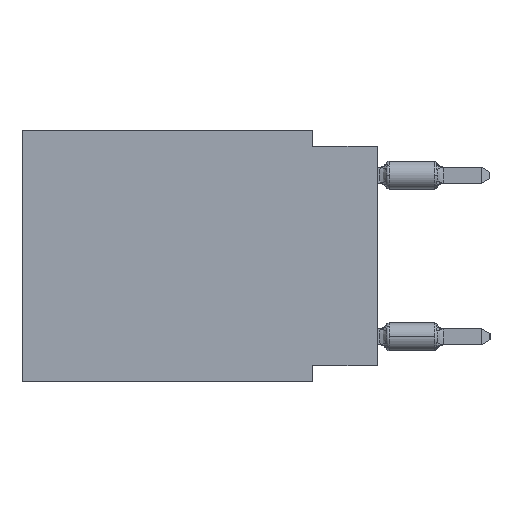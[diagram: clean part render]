
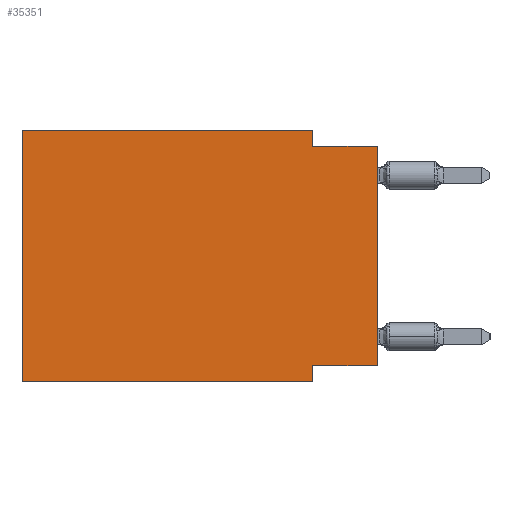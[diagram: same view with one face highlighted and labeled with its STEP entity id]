
A CAD part, left-side view. The second image highlights one B-rep face of the part: STEP entity #35351.
In plain terms, the highlighted planar face has unit normal (-1, 0, 0).
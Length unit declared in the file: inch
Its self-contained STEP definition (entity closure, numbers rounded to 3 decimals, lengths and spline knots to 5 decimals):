
#899 = DIRECTION ( 'NONE',  ( 0., 0., -1. ) ) ;
#2183 = DIRECTION ( 'NONE',  ( 0., 1., 0. ) ) ;
#2944 = VECTOR ( 'NONE', #31111, 39.37008 ) ;
#4536 = VECTOR ( 'NONE', #25142, 39.37008 ) ;
#6134 = LINE ( 'NONE', #20102, #6887 ) ;
#6887 = VECTOR ( 'NONE', #24393, 39.37008 ) ;
#7057 = DIRECTION ( 'NONE',  ( 0., 0., -1. ) ) ;
#7700 = EDGE_CURVE ( 'NONE', #34435, #14014, #41277, .T. ) ;
#8579 = LINE ( 'NONE', #44273, #15129 ) ;
#8936 = CARTESIAN_POINT ( 'NONE',  ( 0., 0., -0.025 ) ) ;
#9552 = VERTEX_POINT ( 'NONE', #8936 ) ;
#10720 = ORIENTED_EDGE ( 'NONE', *, *, #49276, .F. ) ;
#11265 = CARTESIAN_POINT ( 'NONE',  ( 0., 0.1, -0.39 ) ) ;
#11672 = ORIENTED_EDGE ( 'NONE', *, *, #25732, .F. ) ;
#13437 = DIRECTION ( 'NONE',  ( 0., 0., 1. ) ) ;
#13472 = VERTEX_POINT ( 'NONE', #50496 ) ;
#14014 = VERTEX_POINT ( 'NONE', #34338 ) ;
#14554 = CARTESIAN_POINT ( 'NONE',  ( 0., 0.1, 0. ) ) ;
#14652 = LINE ( 'NONE', #14939, #45044 ) ;
#14939 = CARTESIAN_POINT ( 'NONE',  ( 0., 0.55, 0. ) ) ;
#15129 = VECTOR ( 'NONE', #13437, 39.37008 ) ;
#16832 = EDGE_CURVE ( 'NONE', #50899, #9552, #43692, .T. ) ;
#17279 = CARTESIAN_POINT ( 'NONE',  ( 0., 0., -0.365 ) ) ;
#18030 = ORIENTED_EDGE ( 'NONE', *, *, #16832, .F. ) ;
#18857 = DIRECTION ( 'NONE',  ( 1., 0., 0. ) ) ;
#19346 = LINE ( 'NONE', #41317, #32634 ) ;
#20102 = CARTESIAN_POINT ( 'NONE',  ( 0., 0.55, -0.39 ) ) ;
#20781 = EDGE_CURVE ( 'NONE', #14014, #44164, #45247, .T. ) ;
#24393 = DIRECTION ( 'NONE',  ( 0., -1., 0. ) ) ;
#25142 = DIRECTION ( 'NONE',  ( 0., -1., 0. ) ) ;
#25732 = EDGE_CURVE ( 'NONE', #26179, #13472, #44253, .T. ) ;
#25902 = CARTESIAN_POINT ( 'NONE',  ( 0., 0.55, -0.39 ) ) ;
#26179 = VERTEX_POINT ( 'NONE', #25902 ) ;
#27978 = FACE_OUTER_BOUND ( 'NONE', #42163, .T. ) ;
#28060 = DIRECTION ( 'NONE',  ( 0., -1., 0. ) ) ;
#28321 = EDGE_CURVE ( 'NONE', #13472, #35014, #14652, .T. ) ;
#28383 = DIRECTION ( 'NONE',  ( 0., 0., -1. ) ) ;
#28717 = CARTESIAN_POINT ( 'NONE',  ( 0., 0., -0.365 ) ) ;
#29780 = VECTOR ( 'NONE', #2183, 39.37008 ) ;
#31111 = DIRECTION ( 'NONE',  ( 0., 0., 1. ) ) ;
#32634 = VECTOR ( 'NONE', #7057, 39.37008 ) ;
#33953 = ORIENTED_EDGE ( 'NONE', *, *, #44133, .T. ) ;
#34338 = CARTESIAN_POINT ( 'NONE',  ( 0., 0.1, -0.365 ) ) ;
#34435 = VERTEX_POINT ( 'NONE', #17279 ) ;
#35014 = VERTEX_POINT ( 'NONE', #14554 ) ;
#35085 = ORIENTED_EDGE ( 'NONE', *, *, #20781, .F. ) ;
#35351 = ADVANCED_FACE ( 'NONE', ( #27978 ), #44285, .F. ) ;
#38697 = ORIENTED_EDGE ( 'NONE', *, *, #28321, .F. ) ;
#39108 = CARTESIAN_POINT ( 'NONE',  ( 0., 0., -0.025 ) ) ;
#39665 = CARTESIAN_POINT ( 'NONE',  ( 0., 0.55, 0. ) ) ;
#40264 = CARTESIAN_POINT ( 'NONE',  ( 0., 0.55, 0. ) ) ;
#41277 = LINE ( 'NONE', #28717, #29780 ) ;
#41317 = CARTESIAN_POINT ( 'NONE',  ( 0., 0.1, 0. ) ) ;
#42163 = EDGE_LOOP ( 'NONE', ( #48855, #18030, #10720, #38697, #11672, #33953, #35085, #55860 ) ) ;
#43692 = LINE ( 'NONE', #39108, #4536 ) ;
#44133 = EDGE_CURVE ( 'NONE', #26179, #44164, #6134, .T. ) ;
#44164 = VERTEX_POINT ( 'NONE', #11265 ) ;
#44253 = LINE ( 'NONE', #39665, #2944 ) ;
#44273 = CARTESIAN_POINT ( 'NONE',  ( 0., 0., 0. ) ) ;
#44285 = PLANE ( 'NONE',  #53639 ) ;
#44840 = EDGE_CURVE ( 'NONE', #34435, #9552, #8579, .T. ) ;
#45044 = VECTOR ( 'NONE', #28060, 39.37008 ) ;
#45247 = LINE ( 'NONE', #49802, #45771 ) ;
#45771 = VECTOR ( 'NONE', #28383, 39.37008 ) ;
#48855 = ORIENTED_EDGE ( 'NONE', *, *, #44840, .T. ) ;
#49276 = EDGE_CURVE ( 'NONE', #35014, #50899, #19346, .T. ) ;
#49802 = CARTESIAN_POINT ( 'NONE',  ( 0., 0.1, -0.39 ) ) ;
#50496 = CARTESIAN_POINT ( 'NONE',  ( 0., 0.55, 0. ) ) ;
#50641 = CARTESIAN_POINT ( 'NONE',  ( 0., 0.1, -0.025 ) ) ;
#50899 = VERTEX_POINT ( 'NONE', #50641 ) ;
#53639 = AXIS2_PLACEMENT_3D ( 'NONE', #40264, #18857, #899 ) ;
#55860 = ORIENTED_EDGE ( 'NONE', *, *, #7700, .F. ) ;
